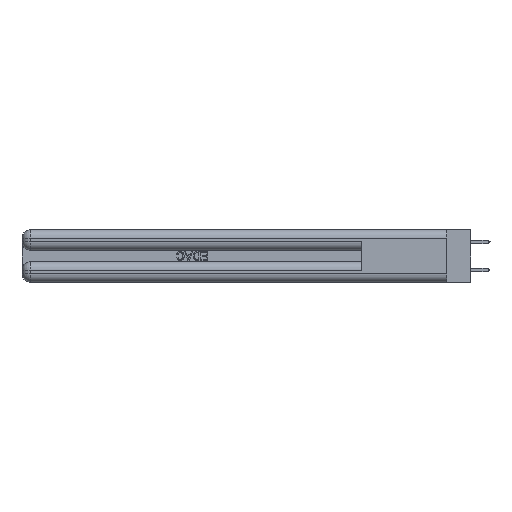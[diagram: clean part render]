
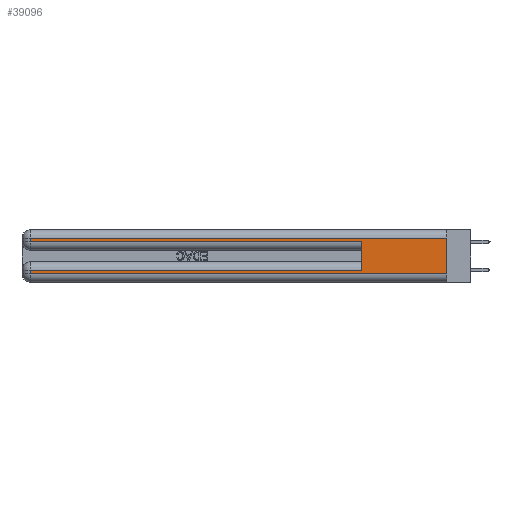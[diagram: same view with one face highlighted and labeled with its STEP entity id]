
A CAD part, left-side view. The second image highlights one B-rep face of the part: STEP entity #39096.
In plain terms, the highlighted planar face has unit normal (-1, 0, 0).
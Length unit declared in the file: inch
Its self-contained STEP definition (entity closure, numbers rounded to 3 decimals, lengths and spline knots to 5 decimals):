
#451 = EDGE_LOOP ( 'NONE', ( #13090, #40255, #32701, #32859, #6320, #27959, #13883, #11773 ) ) ;
#509 = CARTESIAN_POINT ( 'NONE',  ( 0., 0.6, 0.285 ) ) ;
#1606 = CARTESIAN_POINT ( 'NONE',  ( 0., 2.94, 0.085 ) ) ;
#4686 = VECTOR ( 'NONE', #4760, 39.37008 ) ;
#4760 = DIRECTION ( 'NONE',  ( 0., 0., -1. ) ) ;
#5076 = PLANE ( 'NONE',  #6054 ) ;
#5362 = VECTOR ( 'NONE', #13911, 39.37008 ) ;
#6054 = AXIS2_PLACEMENT_3D ( 'NONE', #22617, #22463, #29297 ) ;
#6186 = VERTEX_POINT ( 'NONE', #29875 ) ;
#6320 = ORIENTED_EDGE ( 'NONE', *, *, #32348, .F. ) ;
#6984 = DIRECTION ( 'NONE',  ( 0., 1., 0. ) ) ;
#10506 = CARTESIAN_POINT ( 'NONE',  ( 0., 0., 0.06 ) ) ;
#11451 = DIRECTION ( 'NONE',  ( 0., 1., 0. ) ) ;
#11773 = ORIENTED_EDGE ( 'NONE', *, *, #41331, .T. ) ;
#11789 = LINE ( 'NONE', #10506, #32966 ) ;
#11937 = CARTESIAN_POINT ( 'NONE',  ( 0., 0.6, 0.085 ) ) ;
#12304 = EDGE_CURVE ( 'NONE', #17933, #22224, #37574, .T. ) ;
#12491 = EDGE_CURVE ( 'NONE', #33515, #29064, #19777, .T. ) ;
#13090 = ORIENTED_EDGE ( 'NONE', *, *, #24885, .F. ) ;
#13443 = DIRECTION ( 'NONE',  ( 0., 0., -1. ) ) ;
#13611 = CARTESIAN_POINT ( 'NONE',  ( 0., 2.94, 0.37 ) ) ;
#13883 = ORIENTED_EDGE ( 'NONE', *, *, #32922, .T. ) ;
#13911 = DIRECTION ( 'NONE',  ( 0., 0., 1. ) ) ;
#14982 = CARTESIAN_POINT ( 'NONE',  ( 0., 2.94, 0.31 ) ) ;
#15081 = EDGE_CURVE ( 'NONE', #19525, #33515, #43708, .T. ) ;
#17141 = DIRECTION ( 'NONE',  ( 0., -1., 0. ) ) ;
#17312 = DIRECTION ( 'NONE',  ( 0., 0., -1. ) ) ;
#17870 = CARTESIAN_POINT ( 'NONE',  ( 0., 0.6, 0.145 ) ) ;
#17933 = VERTEX_POINT ( 'NONE', #11937 ) ;
#18095 = EDGE_CURVE ( 'NONE', #6186, #19525, #41202, .T. ) ;
#19525 = VERTEX_POINT ( 'NONE', #14982 ) ;
#19777 = LINE ( 'NONE', #33212, #23044 ) ;
#19861 = CARTESIAN_POINT ( 'NONE',  ( 0., 2.94, 0.06 ) ) ;
#20216 = FACE_OUTER_BOUND ( 'NONE', #451, .T. ) ;
#20682 = VERTEX_POINT ( 'NONE', #19861 ) ;
#22224 = VERTEX_POINT ( 'NONE', #1606 ) ;
#22463 = DIRECTION ( 'NONE',  ( 1., 0., 0. ) ) ;
#22617 = CARTESIAN_POINT ( 'NONE',  ( 0., 0., 0.37 ) ) ;
#23010 = VERTEX_POINT ( 'NONE', #30192 ) ;
#23044 = VECTOR ( 'NONE', #17141, 39.37008 ) ;
#24482 = CARTESIAN_POINT ( 'NONE',  ( 0., 2.94, 0.285 ) ) ;
#24885 = EDGE_CURVE ( 'NONE', #6186, #23010, #38922, .T. ) ;
#27959 = ORIENTED_EDGE ( 'NONE', *, *, #12304, .T. ) ;
#28634 = LINE ( 'NONE', #17870, #5362 ) ;
#29064 = VERTEX_POINT ( 'NONE', #509 ) ;
#29297 = DIRECTION ( 'NONE',  ( 0., 0., -1. ) ) ;
#29354 = VECTOR ( 'NONE', #11451, 39.37008 ) ;
#29875 = CARTESIAN_POINT ( 'NONE',  ( 0., 0., 0.31 ) ) ;
#30192 = CARTESIAN_POINT ( 'NONE',  ( 0., 0., 0.06 ) ) ;
#30764 = VECTOR ( 'NONE', #13443, 39.37008 ) ;
#31342 = CARTESIAN_POINT ( 'NONE',  ( 0., 0., 0.085 ) ) ;
#32348 = EDGE_CURVE ( 'NONE', #17933, #29064, #28634, .T. ) ;
#32701 = ORIENTED_EDGE ( 'NONE', *, *, #15081, .T. ) ;
#32859 = ORIENTED_EDGE ( 'NONE', *, *, #12491, .T. ) ;
#32922 = EDGE_CURVE ( 'NONE', #22224, #20682, #32928, .T. ) ;
#32928 = LINE ( 'NONE', #13611, #30764 ) ;
#32966 = VECTOR ( 'NONE', #42316, 39.37008 ) ;
#33212 = CARTESIAN_POINT ( 'NONE',  ( 0., 0., 0.285 ) ) ;
#33515 = VERTEX_POINT ( 'NONE', #24482 ) ;
#35544 = CARTESIAN_POINT ( 'NONE',  ( 0., 0., 0.31 ) ) ;
#35928 = VECTOR ( 'NONE', #6984, 39.37008 ) ;
#37574 = LINE ( 'NONE', #31342, #35928 ) ;
#38922 = LINE ( 'NONE', #41223, #44400 ) ;
#39096 = ADVANCED_FACE ( 'NONE', ( #20216 ), #5076, .F. ) ;
#40255 = ORIENTED_EDGE ( 'NONE', *, *, #18095, .T. ) ;
#40988 = CARTESIAN_POINT ( 'NONE',  ( 0., 2.94, 0.37 ) ) ;
#41202 = LINE ( 'NONE', #35544, #29354 ) ;
#41223 = CARTESIAN_POINT ( 'NONE',  ( 0., 0., 0.37 ) ) ;
#41331 = EDGE_CURVE ( 'NONE', #20682, #23010, #11789, .T. ) ;
#42316 = DIRECTION ( 'NONE',  ( 0., -1., 0. ) ) ;
#43708 = LINE ( 'NONE', #40988, #4686 ) ;
#44400 = VECTOR ( 'NONE', #17312, 39.37008 ) ;
